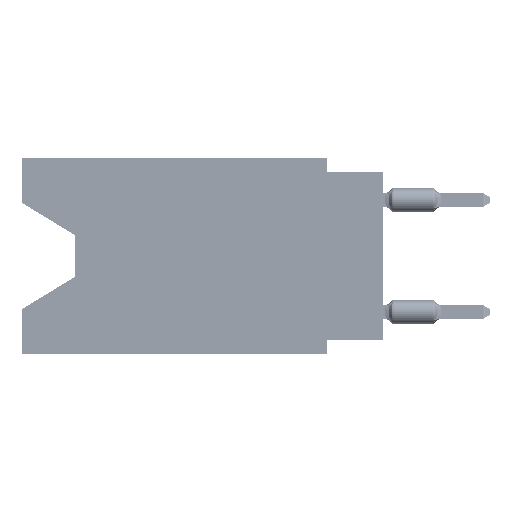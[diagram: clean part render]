
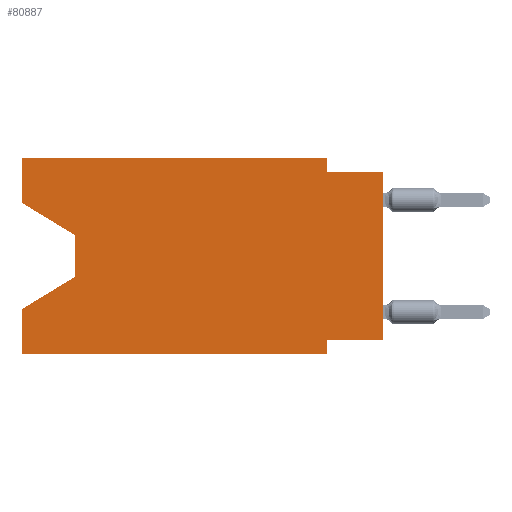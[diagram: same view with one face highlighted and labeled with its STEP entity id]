
A CAD part, left-side view. The second image highlights one B-rep face of the part: STEP entity #80887.
In plain terms, the highlighted planar face has unit normal (-1, 0, 0).
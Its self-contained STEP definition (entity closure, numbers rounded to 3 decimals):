
#1138 = DIRECTION ( 'NONE',  ( 0., 0., 1. ) ) ;
#2051 = EDGE_CURVE ( 'NONE', #63980, #39020, #2492, .T. ) ;
#2492 = LINE ( 'NONE', #43136, #52326 ) ;
#4107 = DIRECTION ( 'NONE',  ( 1., 0., 0. ) ) ;
#4838 = DIRECTION ( 'NONE',  ( 0., -1., 0. ) ) ;
#5659 = LINE ( 'NONE', #74295, #64550 ) ;
#7539 = CARTESIAN_POINT ( 'NONE',  ( 0., 2.54, 0. ) ) ;
#7869 = ORIENTED_EDGE ( 'NONE', *, *, #33553, .F. ) ;
#8837 = VECTOR ( 'NONE', #11470, 1000. ) ;
#9662 = VECTOR ( 'NONE', #4838, 1000. ) ;
#9858 = VERTEX_POINT ( 'NONE', #51801 ) ;
#10870 = ORIENTED_EDGE ( 'NONE', *, *, #85193, .F. ) ;
#10935 = CARTESIAN_POINT ( 'NONE',  ( 0., 0., -0.635 ) ) ;
#11338 = DIRECTION ( 'NONE',  ( 0., 0., -1. ) ) ;
#11470 = DIRECTION ( 'NONE',  ( 0., -1., 0. ) ) ;
#12669 = ORIENTED_EDGE ( 'NONE', *, *, #71217, .F. ) ;
#12835 = EDGE_LOOP ( 'NONE', ( #82772, #79091, #50980, #75473, #49147, #12669, #42165, #79279, #10870, #63655, #72410, #7869 ) ) ;
#14477 = EDGE_CURVE ( 'NONE', #34093, #24957, #66702, .T. ) ;
#14538 = LINE ( 'NONE', #42949, #47331 ) ;
#14632 = EDGE_CURVE ( 'NONE', #32159, #9858, #82942, .T. ) ;
#14710 = LINE ( 'NONE', #42225, #65891 ) ;
#17535 = VERTEX_POINT ( 'NONE', #85127 ) ;
#17713 = LINE ( 'NONE', #65563, #48210 ) ;
#17971 = EDGE_CURVE ( 'NONE', #30998, #32159, #40924, .T. ) ;
#19499 = CARTESIAN_POINT ( 'NONE',  ( 0., 2.54, -0.635 ) ) ;
#22852 = DIRECTION ( 'NONE',  ( 0., -1., 0. ) ) ;
#23601 = VECTOR ( 'NONE', #46797, 1000. ) ;
#24957 = VERTEX_POINT ( 'NONE', #7539 ) ;
#26331 = VECTOR ( 'NONE', #68728, 1000. ) ;
#30998 = VERTEX_POINT ( 'NONE', #82129 ) ;
#31256 = DIRECTION ( 'NONE',  ( 0., 1., 0. ) ) ;
#32159 = VERTEX_POINT ( 'NONE', #87575 ) ;
#32829 = CARTESIAN_POINT ( 'NONE',  ( 0., 16.383, -2.038 ) ) ;
#33211 = DIRECTION ( 'NONE',  ( 0., 0., 1. ) ) ;
#33553 = EDGE_CURVE ( 'NONE', #30998, #34093, #66940, .T. ) ;
#34093 = VERTEX_POINT ( 'NONE', #55910 ) ;
#37162 = LINE ( 'NONE', #43025, #80530 ) ;
#37234 = CARTESIAN_POINT ( 'NONE',  ( 0., 0., -0.635 ) ) ;
#38936 = VERTEX_POINT ( 'NONE', #10935 ) ;
#39020 = VERTEX_POINT ( 'NONE', #74559 ) ;
#40214 = VERTEX_POINT ( 'NONE', #19499 ) ;
#40924 = LINE ( 'NONE', #32829, #23601 ) ;
#42165 = ORIENTED_EDGE ( 'NONE', *, *, #88549, .F. ) ;
#42225 = CARTESIAN_POINT ( 'NONE',  ( 0., 0., 0. ) ) ;
#42949 = CARTESIAN_POINT ( 'NONE',  ( 0., 13.97, -5.385 ) ) ;
#43025 = CARTESIAN_POINT ( 'NONE',  ( 0., 2.54, -8.89 ) ) ;
#43136 = CARTESIAN_POINT ( 'NONE',  ( 0., 16.383, -8.89 ) ) ;
#46797 = DIRECTION ( 'NONE',  ( 0., -0.855, -0.519 ) ) ;
#47331 = VECTOR ( 'NONE', #70501, 1000. ) ;
#48210 = VECTOR ( 'NONE', #31256, 1000. ) ;
#49147 = ORIENTED_EDGE ( 'NONE', *, *, #2051, .T. ) ;
#50980 = ORIENTED_EDGE ( 'NONE', *, *, #52195, .T. ) ;
#51316 = EDGE_CURVE ( 'NONE', #63980, #17535, #5659, .T. ) ;
#51801 = CARTESIAN_POINT ( 'NONE',  ( 0., 13.97, -5.385 ) ) ;
#52195 = EDGE_CURVE ( 'NONE', #9858, #17535, #14538, .T. ) ;
#52263 = VECTOR ( 'NONE', #66312, 1000. ) ;
#52326 = VECTOR ( 'NONE', #22852, 1000. ) ;
#53095 = VERTEX_POINT ( 'NONE', #68516 ) ;
#54091 = CARTESIAN_POINT ( 'NONE',  ( 0., 16.383, -8.89 ) ) ;
#55910 = CARTESIAN_POINT ( 'NONE',  ( 0., 16.383, 0. ) ) ;
#56555 = CARTESIAN_POINT ( 'NONE',  ( 0., 0., -8.255 ) ) ;
#59524 = CARTESIAN_POINT ( 'NONE',  ( 0., 2.54, 0. ) ) ;
#61264 = DIRECTION ( 'NONE',  ( 0., 0., -1. ) ) ;
#62821 = EDGE_CURVE ( 'NONE', #24957, #40214, #86622, .T. ) ;
#63655 = ORIENTED_EDGE ( 'NONE', *, *, #62821, .F. ) ;
#63980 = VERTEX_POINT ( 'NONE', #54091 ) ;
#64550 = VECTOR ( 'NONE', #33211, 1000. ) ;
#64699 = DIRECTION ( 'NONE',  ( 0., 0., -1. ) ) ;
#65563 = CARTESIAN_POINT ( 'NONE',  ( 0., 0., -8.255 ) ) ;
#65891 = VECTOR ( 'NONE', #1138, 1000. ) ;
#65973 = CARTESIAN_POINT ( 'NONE',  ( 0., 16.383, 0. ) ) ;
#66258 = CARTESIAN_POINT ( 'NONE',  ( 0., 16.383, 0. ) ) ;
#66312 = DIRECTION ( 'NONE',  ( 0., 0., -1. ) ) ;
#66702 = LINE ( 'NONE', #66258, #9662 ) ;
#66940 = LINE ( 'NONE', #75035, #26331 ) ;
#67354 = VECTOR ( 'NONE', #61264, 1000. ) ;
#68516 = CARTESIAN_POINT ( 'NONE',  ( 0., 2.54, -8.255 ) ) ;
#68728 = DIRECTION ( 'NONE',  ( 0., 0., 1. ) ) ;
#69552 = EDGE_CURVE ( 'NONE', #88392, #38936, #14710, .T. ) ;
#70501 = DIRECTION ( 'NONE',  ( 0., 0.855, -0.519 ) ) ;
#71217 = EDGE_CURVE ( 'NONE', #53095, #39020, #37162, .T. ) ;
#72410 = ORIENTED_EDGE ( 'NONE', *, *, #14477, .F. ) ;
#73194 = PLANE ( 'NONE',  #74231 ) ;
#73329 = LINE ( 'NONE', #37234, #8837 ) ;
#74231 = AXIS2_PLACEMENT_3D ( 'NONE', #65973, #4107, #11338 ) ;
#74295 = CARTESIAN_POINT ( 'NONE',  ( 0., 16.383, 0. ) ) ;
#74559 = CARTESIAN_POINT ( 'NONE',  ( 0., 2.54, -8.89 ) ) ;
#75035 = CARTESIAN_POINT ( 'NONE',  ( 0., 16.383, 0. ) ) ;
#75256 = CARTESIAN_POINT ( 'NONE',  ( 0., 13.97, -3.505 ) ) ;
#75473 = ORIENTED_EDGE ( 'NONE', *, *, #51316, .F. ) ;
#78634 = FACE_OUTER_BOUND ( 'NONE', #12835, .T. ) ;
#79091 = ORIENTED_EDGE ( 'NONE', *, *, #14632, .T. ) ;
#79279 = ORIENTED_EDGE ( 'NONE', *, *, #69552, .T. ) ;
#80530 = VECTOR ( 'NONE', #64699, 1000. ) ;
#80887 = ADVANCED_FACE ( 'NONE', ( #78634 ), #73194, .F. ) ;
#82129 = CARTESIAN_POINT ( 'NONE',  ( 0., 16.383, -2.038 ) ) ;
#82772 = ORIENTED_EDGE ( 'NONE', *, *, #17971, .T. ) ;
#82942 = LINE ( 'NONE', #75256, #67354 ) ;
#85127 = CARTESIAN_POINT ( 'NONE',  ( 0., 16.383, -6.852 ) ) ;
#85193 = EDGE_CURVE ( 'NONE', #40214, #38936, #73329, .T. ) ;
#86622 = LINE ( 'NONE', #59524, #52263 ) ;
#87575 = CARTESIAN_POINT ( 'NONE',  ( 0., 13.97, -3.505 ) ) ;
#88392 = VERTEX_POINT ( 'NONE', #56555 ) ;
#88549 = EDGE_CURVE ( 'NONE', #88392, #53095, #17713, .T. ) ;
